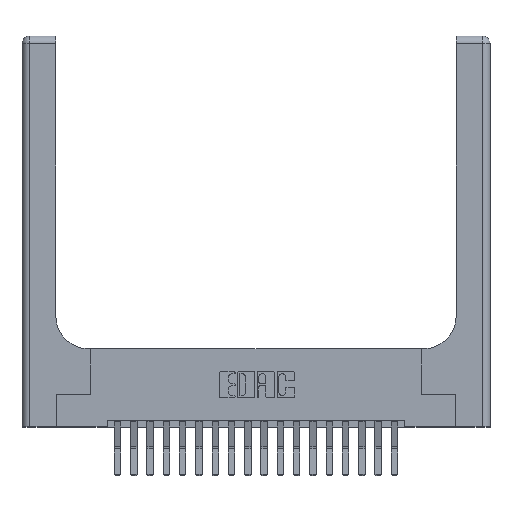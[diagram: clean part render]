
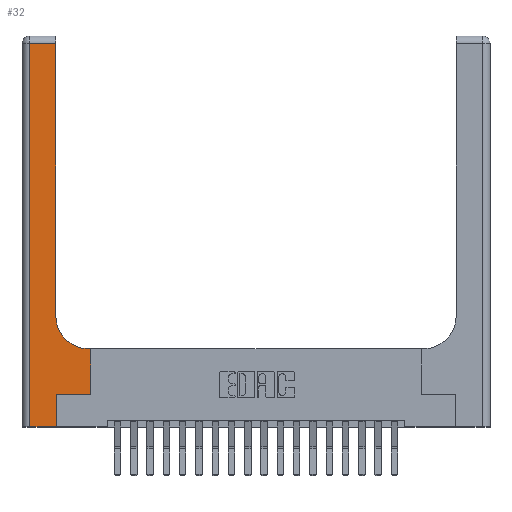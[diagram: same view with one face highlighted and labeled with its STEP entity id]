
A CAD part, top view. The second image highlights one B-rep face of the part: STEP entity #32.
In plain terms, the highlighted planar face has unit normal (0, 0, 1).
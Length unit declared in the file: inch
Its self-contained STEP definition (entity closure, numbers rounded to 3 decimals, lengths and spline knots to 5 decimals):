
#32 = ADVANCED_FACE ( 'NONE', ( #131 ), #8656, .F. ) ;
#76 = ORIENTED_EDGE ( 'NONE', *, *, #11450, .T. ) ;
#131 = FACE_OUTER_BOUND ( 'NONE', #19901, .T. ) ;
#171 = LINE ( 'NONE', #10874, #14357 ) ;
#550 = ORIENTED_EDGE ( 'NONE', *, *, #14785, .T. ) ;
#1536 = VECTOR ( 'NONE', #11002, 39.37008 ) ;
#1763 = CARTESIAN_POINT ( 'NONE',  ( 0.528, 0.25, 0.37 ) ) ;
#2119 = ORIENTED_EDGE ( 'NONE', *, *, #16051, .T. ) ;
#2140 = VERTEX_POINT ( 'NONE', #3605 ) ;
#2167 = CARTESIAN_POINT ( 'NONE',  ( 0.265, 0., 0.37 ) ) ;
#2259 = DIRECTION ( 'NONE',  ( -1., 0., 0. ) ) ;
#3295 = CARTESIAN_POINT ( 'NONE',  ( 0.265, 0., 0.37 ) ) ;
#3605 = CARTESIAN_POINT ( 'NONE',  ( 0.26, 0.85, 0.37 ) ) ;
#3750 = VECTOR ( 'NONE', #2259, 39.37008 ) ;
#4027 = VECTOR ( 'NONE', #15067, 39.37008 ) ;
#4647 = ORIENTED_EDGE ( 'NONE', *, *, #8166, .T. ) ;
#4997 = VERTEX_POINT ( 'NONE', #9260 ) ;
#5110 = ORIENTED_EDGE ( 'NONE', *, *, #16071, .T. ) ;
#5270 = AXIS2_PLACEMENT_3D ( 'NONE', #14727, #14586, #14522 ) ;
#5401 = VERTEX_POINT ( 'NONE', #14663 ) ;
#5518 = ORIENTED_EDGE ( 'NONE', *, *, #15821, .T. ) ;
#5853 = CARTESIAN_POINT ( 'NONE',  ( 0.528, 0.6, 0.37 ) ) ;
#6552 = VERTEX_POINT ( 'NONE', #12147 ) ;
#7193 = CARTESIAN_POINT ( 'NONE',  ( 0.06, 0., 0.37 ) ) ;
#7481 = VERTEX_POINT ( 'NONE', #5853 ) ;
#7681 = EDGE_CURVE ( 'NONE', #12443, #2140, #15350, .T. ) ;
#7879 = DIRECTION ( 'NONE',  ( 1., 0., 0. ) ) ;
#7915 = LINE ( 'NONE', #14689, #3750 ) ;
#8166 = EDGE_CURVE ( 'NONE', #13762, #5401, #19751, .T. ) ;
#8378 = VECTOR ( 'NONE', #7879, 39.37008 ) ;
#8429 = DIRECTION ( 'NONE',  ( -1., 0., 0. ) ) ;
#8458 = LINE ( 'NONE', #13440, #4027 ) ;
#8634 = LINE ( 'NONE', #17226, #8378 ) ;
#8656 = PLANE ( 'NONE',  #11890 ) ;
#9260 = CARTESIAN_POINT ( 'NONE',  ( 0.26, 2.94, 0.37 ) ) ;
#9381 = CARTESIAN_POINT ( 'NONE',  ( 0.528, 0.25, 0.37 ) ) ;
#10226 = DIRECTION ( 'NONE',  ( -1., 0., 0. ) ) ;
#10754 = ORIENTED_EDGE ( 'NONE', *, *, #16595, .T. ) ;
#10844 = LINE ( 'NONE', #17337, #1536 ) ;
#10874 = CARTESIAN_POINT ( 'NONE',  ( 0.26, 3., 0.37 ) ) ;
#11002 = DIRECTION ( 'NONE',  ( 1., 0., 0. ) ) ;
#11450 = EDGE_CURVE ( 'NONE', #7481, #12443, #14967, .T. ) ;
#11890 = AXIS2_PLACEMENT_3D ( 'NONE', #19570, #13221, #10226 ) ;
#12147 = CARTESIAN_POINT ( 'NONE',  ( 0.06, 2.94, 0.37 ) ) ;
#12443 = VERTEX_POINT ( 'NONE', #18327 ) ;
#12450 = DIRECTION ( 'NONE',  ( 0., 1., 0. ) ) ;
#12671 = VECTOR ( 'NONE', #20188, 39.37008 ) ;
#12705 = DIRECTION ( 'NONE',  ( 0., 1., 0. ) ) ;
#13015 = VERTEX_POINT ( 'NONE', #9381 ) ;
#13221 = DIRECTION ( 'NONE',  ( 0., 0., -1. ) ) ;
#13440 = CARTESIAN_POINT ( 'NONE',  ( 0.06, 3., 0.37 ) ) ;
#13502 = EDGE_CURVE ( 'NONE', #2140, #4997, #171, .T. ) ;
#13762 = VERTEX_POINT ( 'NONE', #2167 ) ;
#14353 = ORIENTED_EDGE ( 'NONE', *, *, #13502, .T. ) ;
#14357 = VECTOR ( 'NONE', #12450, 39.37008 ) ;
#14522 = DIRECTION ( 'NONE',  ( 1., 0., 0. ) ) ;
#14586 = DIRECTION ( 'NONE',  ( 0., 0., -1. ) ) ;
#14663 = CARTESIAN_POINT ( 'NONE',  ( 0.265, 0.25, 0.37 ) ) ;
#14689 = CARTESIAN_POINT ( 'NONE',  ( 0., 2.94, 0.37 ) ) ;
#14727 = CARTESIAN_POINT ( 'NONE',  ( 0.51, 0.85, 0.37 ) ) ;
#14785 = EDGE_CURVE ( 'NONE', #6552, #18074, #8458, .T. ) ;
#14967 = LINE ( 'NONE', #17851, #19378 ) ;
#14979 = VECTOR ( 'NONE', #12705, 39.37008 ) ;
#15067 = DIRECTION ( 'NONE',  ( 0., -1., 0. ) ) ;
#15350 = CIRCLE ( 'NONE', #5270, 0.25 ) ;
#15821 = EDGE_CURVE ( 'NONE', #4997, #6552, #7915, .T. ) ;
#16051 = EDGE_CURVE ( 'NONE', #13015, #7481, #18166, .T. ) ;
#16071 = EDGE_CURVE ( 'NONE', #18074, #13762, #10844, .T. ) ;
#16595 = EDGE_CURVE ( 'NONE', #5401, #13015, #8634, .T. ) ;
#17226 = CARTESIAN_POINT ( 'NONE',  ( 0.265, 0.25, 0.37 ) ) ;
#17337 = CARTESIAN_POINT ( 'NONE',  ( 0., 0., 0.37 ) ) ;
#17851 = CARTESIAN_POINT ( 'NONE',  ( 0.26, 0.6, 0.37 ) ) ;
#18074 = VERTEX_POINT ( 'NONE', #7193 ) ;
#18166 = LINE ( 'NONE', #1763, #14979 ) ;
#18327 = CARTESIAN_POINT ( 'NONE',  ( 0.51, 0.6, 0.37 ) ) ;
#19378 = VECTOR ( 'NONE', #8429, 39.37008 ) ;
#19570 = CARTESIAN_POINT ( 'NONE',  ( 0., 3., 0.37 ) ) ;
#19751 = LINE ( 'NONE', #3295, #12671 ) ;
#19901 = EDGE_LOOP ( 'NONE', ( #14353, #5518, #550, #5110, #4647, #10754, #2119, #76, #20065 ) ) ;
#20065 = ORIENTED_EDGE ( 'NONE', *, *, #7681, .T. ) ;
#20188 = DIRECTION ( 'NONE',  ( 0., 1., 0. ) ) ;
